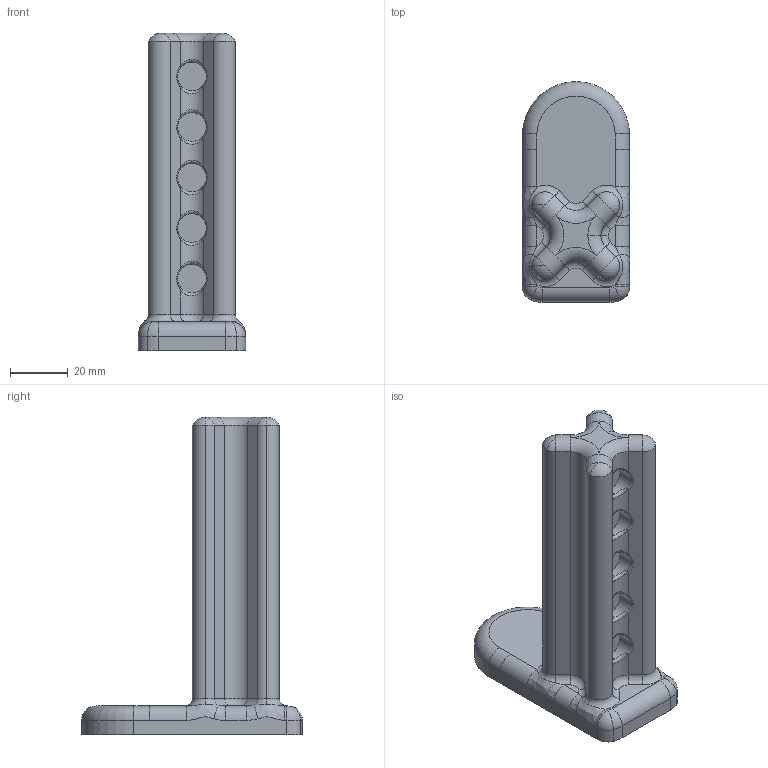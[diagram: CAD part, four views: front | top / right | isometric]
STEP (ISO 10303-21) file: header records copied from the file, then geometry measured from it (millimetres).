
FILE_DESCRIPTION (( 'STEP AP214' ), '1' );
FILE_NAME ('Stock_Arm_V2.STEP', '2013-10-25T16:58:33', ( 'elpi' ), ( '' ), 'SwSTEP 2.0', 'SolidWorks 2013', '' );
FILE_SCHEMA (( 'AUTOMOTIVE_DESIGN' ));
Length unit declared in the file: millimetre
Products named in the file (1): Stock_Arm_V2
Bounding box: 37.13 x 76.47 x 110 mm (x, y, z)
Volume: 84282.9 mm3; surface area: 20743.4 mm2
Topology: 1 solids, 1 shells, 146 faces, 342 edges, 200 vertices
Faces by surface type: cylinder 57, bspline 38, plane 24, torus 19, sphere 8
Entity records: 6191 total; most frequent: CARTESIAN_POINT 3097, ORIENTED_EDGE 684, DIRECTION 625, EDGE_CURVE 342, AXIS2_PLACEMENT_3D 264, VERTEX_POINT 200, CIRCLE 155, EDGE_LOOP 148
